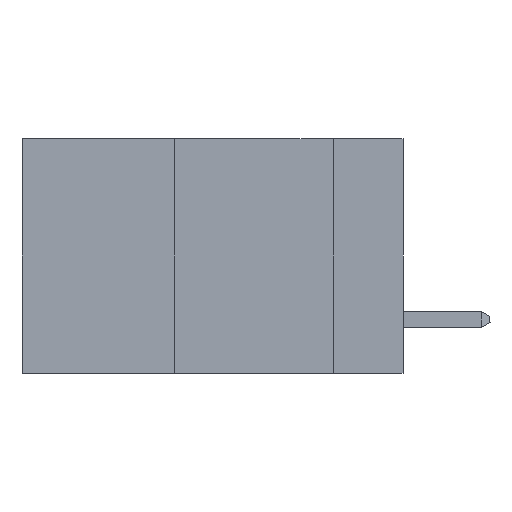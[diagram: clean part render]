
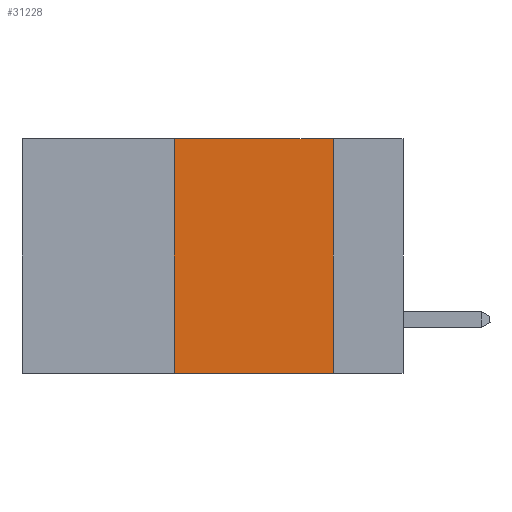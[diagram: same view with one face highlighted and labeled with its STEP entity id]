
A CAD part, left-side view. The second image highlights one B-rep face of the part: STEP entity #31228.
In plain terms, the highlighted planar face has unit normal (-1, 0, 0).
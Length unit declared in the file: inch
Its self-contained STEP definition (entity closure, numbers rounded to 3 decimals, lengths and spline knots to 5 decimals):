
#1924 = LINE ( 'NONE', #31721, #20573 ) ;
#1979 = EDGE_LOOP ( 'NONE', ( #14784, #30158, #18958, #14277 ) ) ;
#2403 = EDGE_CURVE ( 'NONE', #11446, #18455, #12130, .T. ) ;
#2792 = EDGE_CURVE ( 'NONE', #11446, #28001, #1924, .T. ) ;
#3605 = CARTESIAN_POINT ( 'NONE',  ( 0., 0.6, 0. ) ) ;
#4706 = VECTOR ( 'NONE', #23578, 39.37008 ) ;
#5372 = DIRECTION ( 'NONE',  ( 1., 0., 0. ) ) ;
#5569 = CARTESIAN_POINT ( 'NONE',  ( 0., 0.6, 0. ) ) ;
#5802 = VECTOR ( 'NONE', #14032, 39.37008 ) ;
#7234 = CARTESIAN_POINT ( 'NONE',  ( 0., 0.36, 0. ) ) ;
#7385 = VECTOR ( 'NONE', #29542, 39.37008 ) ;
#7770 = DIRECTION ( 'NONE',  ( 0., 0., -1. ) ) ;
#10774 = EDGE_CURVE ( 'NONE', #21869, #28001, #30844, .T. ) ;
#10850 = AXIS2_PLACEMENT_3D ( 'NONE', #5569, #5372, #7770 ) ;
#11446 = VERTEX_POINT ( 'NONE', #13144 ) ;
#11920 = DIRECTION ( 'NONE',  ( 0., -1., 0. ) ) ;
#12130 = LINE ( 'NONE', #7234, #7385 ) ;
#12150 = LINE ( 'NONE', #3605, #4706 ) ;
#13144 = CARTESIAN_POINT ( 'NONE',  ( 0., 0.36, -0.37 ) ) ;
#14032 = DIRECTION ( 'NONE',  ( 0., 0., -1. ) ) ;
#14277 = ORIENTED_EDGE ( 'NONE', *, *, #2792, .T. ) ;
#14784 = ORIENTED_EDGE ( 'NONE', *, *, #10774, .F. ) ;
#14786 = FACE_OUTER_BOUND ( 'NONE', #1979, .T. ) ;
#15061 = CARTESIAN_POINT ( 'NONE',  ( 0., 0.11, -0.37 ) ) ;
#17738 = EDGE_CURVE ( 'NONE', #18455, #21869, #12150, .T. ) ;
#18455 = VERTEX_POINT ( 'NONE', #29720 ) ;
#18958 = ORIENTED_EDGE ( 'NONE', *, *, #2403, .F. ) ;
#20503 = PLANE ( 'NONE',  #10850 ) ;
#20540 = CARTESIAN_POINT ( 'NONE',  ( 0., 0.11, 0. ) ) ;
#20573 = VECTOR ( 'NONE', #11920, 39.37008 ) ;
#21869 = VERTEX_POINT ( 'NONE', #20540 ) ;
#23578 = DIRECTION ( 'NONE',  ( 0., -1., 0. ) ) ;
#28001 = VERTEX_POINT ( 'NONE', #15061 ) ;
#29542 = DIRECTION ( 'NONE',  ( 0., 0., 1. ) ) ;
#29720 = CARTESIAN_POINT ( 'NONE',  ( 0., 0.36, 0. ) ) ;
#30158 = ORIENTED_EDGE ( 'NONE', *, *, #17738, .F. ) ;
#30169 = CARTESIAN_POINT ( 'NONE',  ( 0., 0.11, 0. ) ) ;
#30844 = LINE ( 'NONE', #30169, #5802 ) ;
#31228 = ADVANCED_FACE ( 'NONE', ( #14786 ), #20503, .F. ) ;
#31721 = CARTESIAN_POINT ( 'NONE',  ( 0., 0.6, -0.37 ) ) ;
